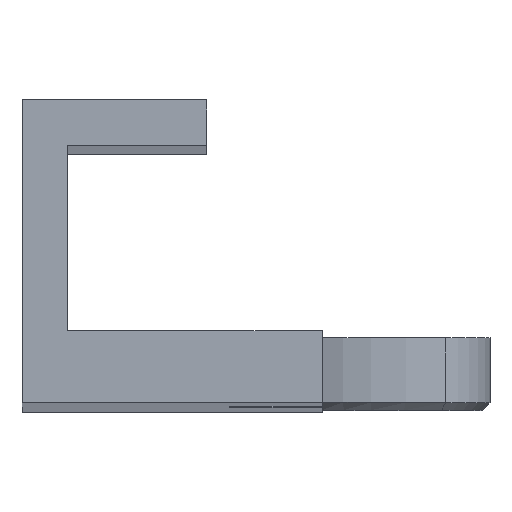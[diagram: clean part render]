
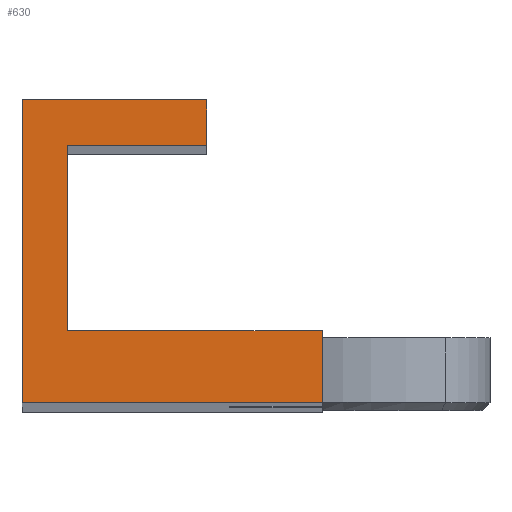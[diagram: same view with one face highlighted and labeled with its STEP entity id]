
A CAD part, top view. The second image highlights one B-rep face of the part: STEP entity #630.
In plain terms, the highlighted planar face has unit normal (0, 0, 1).
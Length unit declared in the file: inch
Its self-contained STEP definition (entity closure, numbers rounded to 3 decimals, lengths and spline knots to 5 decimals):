
#56=FACE_OUTER_BOUND('',#86,.T.);
#86=EDGE_LOOP('',(#486,#487,#488,#489,#490,#491,#492,#493));
#159=LINE('',#935,#218);
#175=LINE('',#979,#234);
#184=LINE('',#995,#243);
#185=LINE('',#998,#244);
#186=LINE('',#1000,#245);
#187=LINE('',#1002,#246);
#188=LINE('',#1004,#247);
#189=LINE('',#1005,#248);
#218=VECTOR('',#745,0.3937);
#234=VECTOR('',#783,0.3937);
#243=VECTOR('',#800,0.3937);
#244=VECTOR('',#803,0.3937);
#245=VECTOR('',#804,0.3937);
#246=VECTOR('',#805,0.3937);
#247=VECTOR('',#806,0.3937);
#248=VECTOR('',#807,0.3937);
#279=VERTEX_POINT('',#932);
#280=VERTEX_POINT('',#934);
#293=VERTEX_POINT('',#976);
#294=VERTEX_POINT('',#978);
#298=VERTEX_POINT('',#997);
#299=VERTEX_POINT('',#999);
#300=VERTEX_POINT('',#1001);
#301=VERTEX_POINT('',#1003);
#341=EDGE_CURVE('',#279,#280,#159,.T.);
#362=EDGE_CURVE('',#293,#294,#175,.T.);
#371=EDGE_CURVE('',#280,#293,#184,.T.);
#372=EDGE_CURVE('',#298,#279,#185,.T.);
#373=EDGE_CURVE('',#299,#298,#186,.T.);
#374=EDGE_CURVE('',#300,#299,#187,.T.);
#375=EDGE_CURVE('',#301,#300,#188,.T.);
#376=EDGE_CURVE('',#294,#301,#189,.T.);
#486=ORIENTED_EDGE('',*,*,#371,.F.);
#487=ORIENTED_EDGE('',*,*,#341,.F.);
#488=ORIENTED_EDGE('',*,*,#372,.F.);
#489=ORIENTED_EDGE('',*,*,#373,.F.);
#490=ORIENTED_EDGE('',*,*,#374,.F.);
#491=ORIENTED_EDGE('',*,*,#375,.F.);
#492=ORIENTED_EDGE('',*,*,#376,.F.);
#493=ORIENTED_EDGE('',*,*,#362,.F.);
#608=PLANE('',#686);
#630=ADVANCED_FACE('',(#56),#608,.F.);
#686=AXIS2_PLACEMENT_3D('',#996,#801,#802);
#745=DIRECTION('',(1.,0.,0.));
#783=DIRECTION('',(-1.,0.,0.));
#800=DIRECTION('',(0.,-1.,0.));
#801=DIRECTION('center_axis',(0.,0.,-1.));
#802=DIRECTION('ref_axis',(-1.,0.,0.));
#803=DIRECTION('',(0.,-1.,0.));
#804=DIRECTION('',(-1.,0.,0.));
#805=DIRECTION('',(0.,-1.,0.));
#806=DIRECTION('',(1.,0.,0.));
#807=DIRECTION('',(0.,1.,0.));
#932=CARTESIAN_POINT('',(-0.33094,0.09406,6.80194));
#934=CARTESIAN_POINT('',(0.,0.09406,6.80194));
#935=CARTESIAN_POINT('',(-0.33094,0.09406,6.80194));
#976=CARTESIAN_POINT('',(0.,0.,6.80194));
#978=CARTESIAN_POINT('',(-0.39,0.,6.80194));
#979=CARTESIAN_POINT('',(-0.2925,0.,6.80194));
#995=CARTESIAN_POINT('',(0.,0.09843,6.80194));
#996=CARTESIAN_POINT('Origin',(-0.195,0.19685,6.80194));
#997=CARTESIAN_POINT('',(-0.33094,0.33465,6.80194));
#998=CARTESIAN_POINT('',(-0.33094,0.12795,6.80194));
#999=CARTESIAN_POINT('',(-0.15,0.33465,6.80194));
#1000=CARTESIAN_POINT('',(-0.26297,0.33465,6.80194));
#1001=CARTESIAN_POINT('',(-0.15,0.3937,6.80194));
#1002=CARTESIAN_POINT('',(-0.15,0.29528,6.80194));
#1003=CARTESIAN_POINT('',(-0.39,0.3937,6.80194));
#1004=CARTESIAN_POINT('',(-0.1525,0.3937,6.80194));
#1005=CARTESIAN_POINT('',(-0.39,0.29528,6.80194));
